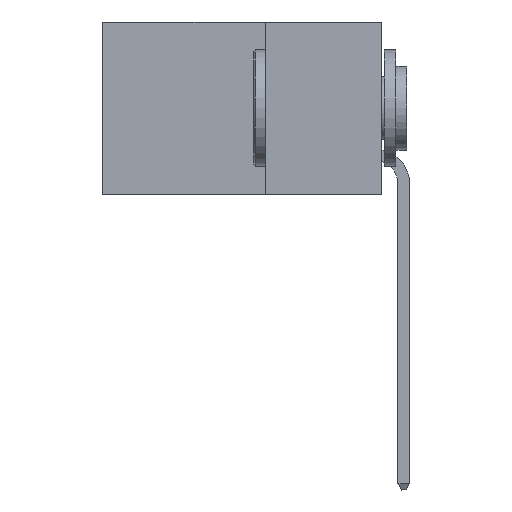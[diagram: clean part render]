
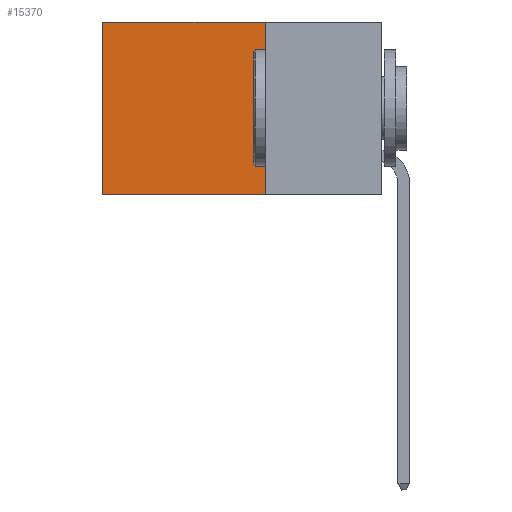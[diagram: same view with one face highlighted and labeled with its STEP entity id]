
A CAD part, left-side view. The second image highlights one B-rep face of the part: STEP entity #15370.
In plain terms, the highlighted planar face has unit normal (-1, 0, 0).
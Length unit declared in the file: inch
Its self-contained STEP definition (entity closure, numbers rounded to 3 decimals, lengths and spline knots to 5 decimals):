
#830 = CARTESIAN_POINT ( 'NONE',  ( 0.2875, 0.6, 0. ) ) ;
#1339 = FACE_OUTER_BOUND ( 'NONE', #25570, .T. ) ;
#2385 = VERTEX_POINT ( 'NONE', #5949 ) ;
#4744 = DIRECTION ( 'NONE',  ( 0., 0., -1. ) ) ;
#4861 = CARTESIAN_POINT ( 'NONE',  ( 0.2875, 0.25, -0.37 ) ) ;
#5678 = CARTESIAN_POINT ( 'NONE',  ( 0.2875, 0.25, 0. ) ) ;
#5949 = CARTESIAN_POINT ( 'NONE',  ( 0.2875, 0.6, -0.37 ) ) ;
#6608 = DIRECTION ( 'NONE',  ( 1., 0., 0. ) ) ;
#6981 = EDGE_CURVE ( 'NONE', #46727, #2385, #17116, .T. ) ;
#9051 = ORIENTED_EDGE ( 'NONE', *, *, #10906, .T. ) ;
#10906 = EDGE_CURVE ( 'NONE', #16835, #46727, #32046, .T. ) ;
#15370 = ADVANCED_FACE ( 'NONE', ( #1339 ), #29305, .F. ) ;
#15766 = AXIS2_PLACEMENT_3D ( 'NONE', #21402, #6608, #25657 ) ;
#16835 = VERTEX_POINT ( 'NONE', #16868 ) ;
#16868 = CARTESIAN_POINT ( 'NONE',  ( 0.2875, 0.25, 0. ) ) ;
#17116 = LINE ( 'NONE', #830, #17728 ) ;
#17728 = VECTOR ( 'NONE', #19261, 39.37008 ) ;
#19261 = DIRECTION ( 'NONE',  ( 0., 0., -1. ) ) ;
#19311 = ORIENTED_EDGE ( 'NONE', *, *, #6981, .T. ) ;
#20297 = CARTESIAN_POINT ( 'NONE',  ( 0.2875, 0.25, -0.37 ) ) ;
#21402 = CARTESIAN_POINT ( 'NONE',  ( 0.2875, 0.25, 0. ) ) ;
#23159 = CARTESIAN_POINT ( 'NONE',  ( 0.2875, 0.25, 0. ) ) ;
#23459 = LINE ( 'NONE', #20297, #26391 ) ;
#25570 = EDGE_LOOP ( 'NONE', ( #19311, #36952, #46606, #9051 ) ) ;
#25657 = DIRECTION ( 'NONE',  ( 0., 0., -1. ) ) ;
#26391 = VECTOR ( 'NONE', #35522, 39.37008 ) ;
#27047 = LINE ( 'NONE', #23159, #47241 ) ;
#29305 = PLANE ( 'NONE',  #15766 ) ;
#31493 = VERTEX_POINT ( 'NONE', #4861 ) ;
#32046 = LINE ( 'NONE', #5678, #37992 ) ;
#33140 = EDGE_CURVE ( 'NONE', #31493, #2385, #23459, .T. ) ;
#35522 = DIRECTION ( 'NONE',  ( 0., 1., 0. ) ) ;
#36952 = ORIENTED_EDGE ( 'NONE', *, *, #33140, .F. ) ;
#37992 = VECTOR ( 'NONE', #43630, 39.37008 ) ;
#38921 = EDGE_CURVE ( 'NONE', #16835, #31493, #27047, .T. ) ;
#41347 = CARTESIAN_POINT ( 'NONE',  ( 0.2875, 0.6, 0. ) ) ;
#43630 = DIRECTION ( 'NONE',  ( 0., 1., 0. ) ) ;
#46606 = ORIENTED_EDGE ( 'NONE', *, *, #38921, .F. ) ;
#46727 = VERTEX_POINT ( 'NONE', #41347 ) ;
#47241 = VECTOR ( 'NONE', #4744, 39.37008 ) ;
